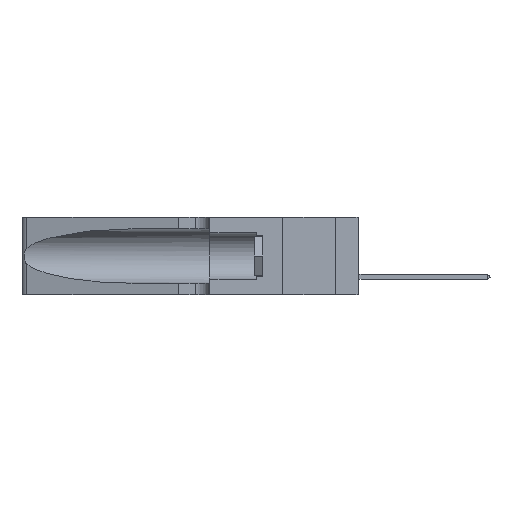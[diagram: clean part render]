
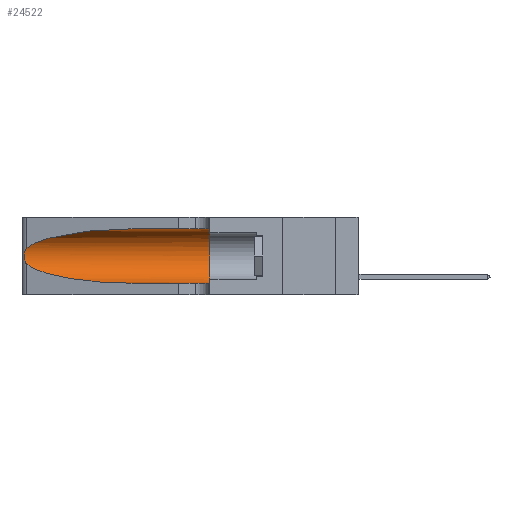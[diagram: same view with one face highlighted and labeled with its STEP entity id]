
A CAD part, left-side view. The second image highlights one B-rep face of the part: STEP entity #24522.
In plain terms, the highlighted cylindrical face has radius 3.308 mm (diameter 6.617 mm), a partial arc.
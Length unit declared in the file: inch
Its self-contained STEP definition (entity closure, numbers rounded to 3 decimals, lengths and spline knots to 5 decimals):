
#404 = VERTEX_POINT ( 'NONE', #8254 ) ;
#518 = CARTESIAN_POINT ( 'NONE',  ( 0.1305, 0.72297, 0.31525 ) ) ;
#661 = ORIENTED_EDGE ( 'NONE', *, *, #5099, .T. ) ;
#692 = ORIENTED_EDGE ( 'NONE', *, *, #31864, .F. ) ;
#1291 = CARTESIAN_POINT ( 'NONE',  ( 0.25487, 1.22718, 0.22369 ) ) ;
#1544 = CARTESIAN_POINT ( 'NONE',  ( 0.2373, 1.15595, 0.08982 ) ) ;
#2322 = CIRCLE ( 'NONE', #19619, 0.13025 ) ;
#4142 = CARTESIAN_POINT ( 'NONE',  ( 0.26075, 1.23896, 0.19203 ) ) ;
#4977 = VECTOR ( 'NONE', #6180, 39.37008 ) ;
#5099 = EDGE_CURVE ( 'NONE', #28180, #6632, #9495, .T. ) ;
#5808 = CARTESIAN_POINT ( 'NONE',  ( 0.25487, 1.22718, 0.14631 ) ) ;
#6180 = DIRECTION ( 'NONE',  ( 0., -1., 0. ) ) ;
#6237 = CARTESIAN_POINT ( 'NONE',  ( 0.1305, 0.35, 0.31525 ) ) ;
#6632 = VERTEX_POINT ( 'NONE', #33878 ) ;
#7157 = CARTESIAN_POINT ( 'NONE',  ( 0.25487, 1.22718, 0.22369 ) ) ;
#8077 = CARTESIAN_POINT ( 'NONE',  ( 0.1305, 1.61858, 0.05475 ) ) ;
#8254 = CARTESIAN_POINT ( 'NONE',  ( 0.1305, 0.35, 0.05475 ) ) ;
#9050 = CARTESIAN_POINT ( 'NONE',  ( 0.26018, 1.23835, 0.19895 ) ) ;
#9266 = CARTESIAN_POINT ( 'NONE',  ( 0.25639, 1.23184, 0.21858 ) ) ;
#9495 =( BOUNDED_CURVE ( )  B_SPLINE_CURVE ( 3, ( #30299, #1544, #19837, #20297 ),
 .UNSPECIFIED., .F., .T. ) 
 B_SPLINE_CURVE_WITH_KNOTS ( ( 4, 4 ),
 ( 3.44316, 4.71239 ),
 .UNSPECIFIED. ) 
 CURVE ( )  GEOMETRIC_REPRESENTATION_ITEM ( )  RATIONAL_B_SPLINE_CURVE ( ( 1., 0.87, 0.87, 1. ) ) 
 REPRESENTATION_ITEM ( '' )  );
#10274 = DIRECTION ( 'NONE',  ( 0., 0., 1. ) ) ;
#10781 = DIRECTION ( 'NONE',  ( 0., -1., 0. ) ) ;
#11869 = CARTESIAN_POINT ( 'NONE',  ( 0.25856, 1.23593, 0.16098 ) ) ;
#12883 = ORIENTED_EDGE ( 'NONE', *, *, #25737, .T. ) ;
#13370 = VERTEX_POINT ( 'NONE', #518 ) ;
#14188 = CARTESIAN_POINT ( 'NONE',  ( 0.2373, 1.15595, 0.28018 ) ) ;
#14538 = CARTESIAN_POINT ( 'NONE',  ( 0.26075, 1.23896, 0.178 ) ) ;
#15530 = EDGE_LOOP ( 'NONE', ( #22332, #12883, #661, #33656, #692, #18196 ) ) ;
#15960 = VECTOR ( 'NONE', #31682, 39.37008 ) ;
#16450 = LINE ( 'NONE', #26826, #4977 ) ;
#17561 = CYLINDRICAL_SURFACE ( 'NONE', #26972, 0.13025 ) ;
#18046 = VERTEX_POINT ( 'NONE', #6237 ) ;
#18196 = ORIENTED_EDGE ( 'NONE', *, *, #22884, .F. ) ;
#18811 = DIRECTION ( 'NONE',  ( 0., 0., -1. ) ) ;
#19619 = AXIS2_PLACEMENT_3D ( 'NONE', #31393, #31068, #10274 ) ;
#19806 = CARTESIAN_POINT ( 'NONE',  ( 0.25639, 1.23186, 0.15144 ) ) ;
#19837 = CARTESIAN_POINT ( 'NONE',  ( 0.18966, 0.96281, 0.05475 ) ) ;
#20297 = CARTESIAN_POINT ( 'NONE',  ( 0.1305, 0.72297, 0.05475 ) ) ;
#21343 = CARTESIAN_POINT ( 'NONE',  ( 0.1305, 1.61858, 0.185 ) ) ;
#21832 = EDGE_CURVE ( 'NONE', #13370, #29377, #25884, .T. ) ;
#21861 = CARTESIAN_POINT ( 'NONE',  ( 0.18966, 0.96281, 0.31525 ) ) ;
#22100 = CARTESIAN_POINT ( 'NONE',  ( 0.25555, 1.22993, 0.14849 ) ) ;
#22214 = CARTESIAN_POINT ( 'NONE',  ( 0.25487, 1.22718, 0.14631 ) ) ;
#22332 = ORIENTED_EDGE ( 'NONE', *, *, #21832, .T. ) ;
#22884 = EDGE_CURVE ( 'NONE', #13370, #18046, #16450, .T. ) ;
#22903 = LINE ( 'NONE', #8077, #15960 ) ;
#24522 = ADVANCED_FACE ( 'NONE', ( #31909 ), #17561, .F. ) ;
#24609 = CARTESIAN_POINT ( 'NONE',  ( 0.26017, 1.23833, 0.17102 ) ) ;
#24953 = CARTESIAN_POINT ( 'NONE',  ( 0.25555, 1.22994, 0.2215 ) ) ;
#25737 = EDGE_CURVE ( 'NONE', #29377, #28180, #27342, .T. ) ;
#25884 =( BOUNDED_CURVE ( )  B_SPLINE_CURVE ( 3, ( #29339, #21861, #14188, #27597 ),
 .UNSPECIFIED., .F., .F. ) 
 B_SPLINE_CURVE_WITH_KNOTS ( ( 4, 4 ),
 ( 1.5708, 2.84003 ),
 .UNSPECIFIED. ) 
 CURVE ( )  GEOMETRIC_REPRESENTATION_ITEM ( )  RATIONAL_B_SPLINE_CURVE ( ( 1., 0.87, 0.87, 1. ) ) 
 REPRESENTATION_ITEM ( '' )  );
#26826 = CARTESIAN_POINT ( 'NONE',  ( 0.1305, 1.61858, 0.31525 ) ) ;
#26972 = AXIS2_PLACEMENT_3D ( 'NONE', #21343, #10781, #18811 ) ;
#27342 = B_SPLINE_CURVE_WITH_KNOTS ( 'NONE', 3,
 ( #1291, #24953, #9266, #30030, #27612, #9050, #4142, #14538, #24609, #11869, #32451, #19806, #22100, #22214 ),
 .UNSPECIFIED., .F., .F.,
 ( 4, 2, 2, 2, 2, 2, 4 ),
 ( 0., 0.00027, 0.00053, 0.00107, 0.0016, 0.00187, 0.00214 ),
 .UNSPECIFIED. ) ;
#27597 = CARTESIAN_POINT ( 'NONE',  ( 0.25487, 1.22718, 0.22369 ) ) ;
#27612 = CARTESIAN_POINT ( 'NONE',  ( 0.25854, 1.2359, 0.20912 ) ) ;
#28180 = VERTEX_POINT ( 'NONE', #5808 ) ;
#29339 = CARTESIAN_POINT ( 'NONE',  ( 0.1305, 0.72297, 0.31525 ) ) ;
#29377 = VERTEX_POINT ( 'NONE', #7157 ) ;
#29690 = EDGE_CURVE ( 'NONE', #6632, #404, #22903, .T. ) ;
#30030 = CARTESIAN_POINT ( 'NONE',  ( 0.25787, 1.23484, 0.2124 ) ) ;
#30299 = CARTESIAN_POINT ( 'NONE',  ( 0.25487, 1.22718, 0.14631 ) ) ;
#31068 = DIRECTION ( 'NONE',  ( 0., 1., 0. ) ) ;
#31393 = CARTESIAN_POINT ( 'NONE',  ( 0.1305, 0.35, 0.185 ) ) ;
#31682 = DIRECTION ( 'NONE',  ( 0., -1., 0. ) ) ;
#31864 = EDGE_CURVE ( 'NONE', #18046, #404, #2322, .T. ) ;
#31909 = FACE_OUTER_BOUND ( 'NONE', #15530, .T. ) ;
#32451 = CARTESIAN_POINT ( 'NONE',  ( 0.25789, 1.23486, 0.15765 ) ) ;
#33656 = ORIENTED_EDGE ( 'NONE', *, *, #29690, .T. ) ;
#33878 = CARTESIAN_POINT ( 'NONE',  ( 0.1305, 0.72297, 0.05475 ) ) ;
